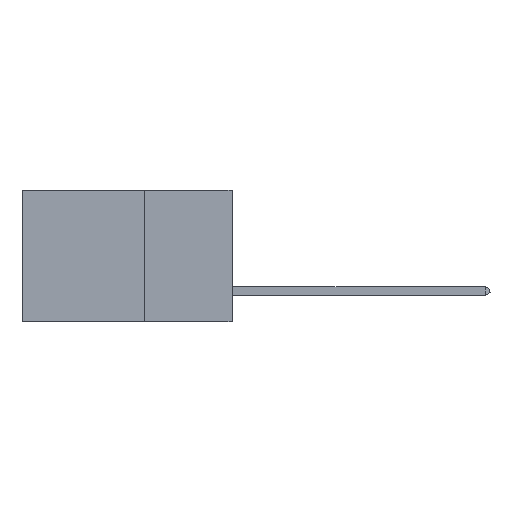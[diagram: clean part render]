
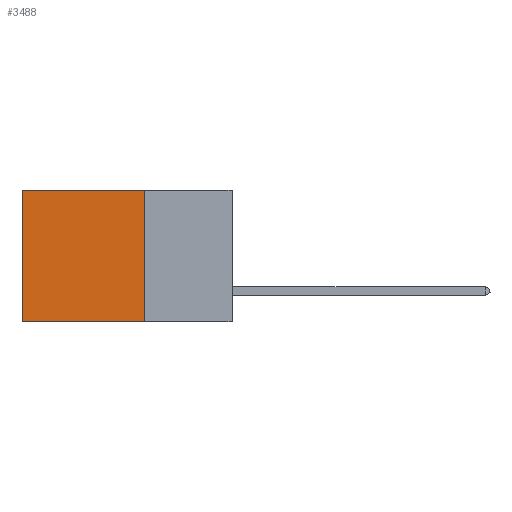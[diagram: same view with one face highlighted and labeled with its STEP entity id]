
A CAD part, left-side view. The second image highlights one B-rep face of the part: STEP entity #3488.
In plain terms, the highlighted planar face has unit normal (-1, 0, 0).
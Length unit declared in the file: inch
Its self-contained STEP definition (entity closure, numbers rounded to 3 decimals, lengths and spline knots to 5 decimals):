
#226 = VECTOR ( 'NONE', #7863, 39.37008 ) ;
#321 = VERTEX_POINT ( 'NONE', #3497 ) ;
#1167 = CARTESIAN_POINT ( 'NONE',  ( 0.2875, 0.25, -0.375 ) ) ;
#1226 = EDGE_CURVE ( 'NONE', #4957, #321, #12450, .T. ) ;
#1494 = LINE ( 'NONE', #4837, #12301 ) ;
#2737 = AXIS2_PLACEMENT_3D ( 'NONE', #10903, #4791, #12801 ) ;
#2870 = EDGE_LOOP ( 'NONE', ( #8699, #11820, #7296, #12057 ) ) ;
#3081 = CARTESIAN_POINT ( 'NONE',  ( 0.2875, 0.25, -0.375 ) ) ;
#3129 = LINE ( 'NONE', #6949, #7801 ) ;
#3488 = ADVANCED_FACE ( 'NONE', ( #8814 ), #9737, .F. ) ;
#3497 = CARTESIAN_POINT ( 'NONE',  ( 0.2875, 0.6, -0.375 ) ) ;
#3560 = CARTESIAN_POINT ( 'NONE',  ( 0.2875, 0.6, 0. ) ) ;
#4108 = EDGE_CURVE ( 'NONE', #10696, #321, #3129, .T. ) ;
#4565 = CARTESIAN_POINT ( 'NONE',  ( 0.2875, 0.25, 0. ) ) ;
#4791 = DIRECTION ( 'NONE',  ( 1., 0., 0. ) ) ;
#4837 = CARTESIAN_POINT ( 'NONE',  ( 0.2875, 0.25, -0.375 ) ) ;
#4957 = VERTEX_POINT ( 'NONE', #3081 ) ;
#5743 = VECTOR ( 'NONE', #9517, 39.37008 ) ;
#6155 = DIRECTION ( 'NONE',  ( 0., 0., -1. ) ) ;
#6812 = LINE ( 'NONE', #12716, #226 ) ;
#6949 = CARTESIAN_POINT ( 'NONE',  ( 0.2875, 0.6, -0.375 ) ) ;
#7296 = ORIENTED_EDGE ( 'NONE', *, *, #12970, .F. ) ;
#7801 = VECTOR ( 'NONE', #6155, 39.37008 ) ;
#7863 = DIRECTION ( 'NONE',  ( 0., 1., 0. ) ) ;
#8699 = ORIENTED_EDGE ( 'NONE', *, *, #4108, .T. ) ;
#8814 = FACE_OUTER_BOUND ( 'NONE', #2870, .T. ) ;
#9517 = DIRECTION ( 'NONE',  ( 0., 1., 0. ) ) ;
#9737 = PLANE ( 'NONE',  #2737 ) ;
#9842 = DIRECTION ( 'NONE',  ( 0., 0., -1. ) ) ;
#9873 = VERTEX_POINT ( 'NONE', #4565 ) ;
#10063 = EDGE_CURVE ( 'NONE', #9873, #10696, #6812, .T. ) ;
#10696 = VERTEX_POINT ( 'NONE', #3560 ) ;
#10903 = CARTESIAN_POINT ( 'NONE',  ( 0.2875, 0.25, -0.375 ) ) ;
#11820 = ORIENTED_EDGE ( 'NONE', *, *, #1226, .F. ) ;
#12057 = ORIENTED_EDGE ( 'NONE', *, *, #10063, .T. ) ;
#12301 = VECTOR ( 'NONE', #9842, 39.37008 ) ;
#12450 = LINE ( 'NONE', #1167, #5743 ) ;
#12716 = CARTESIAN_POINT ( 'NONE',  ( 0.2875, 0.25, 0. ) ) ;
#12801 = DIRECTION ( 'NONE',  ( 0., 0., -1. ) ) ;
#12970 = EDGE_CURVE ( 'NONE', #9873, #4957, #1494, .T. ) ;
